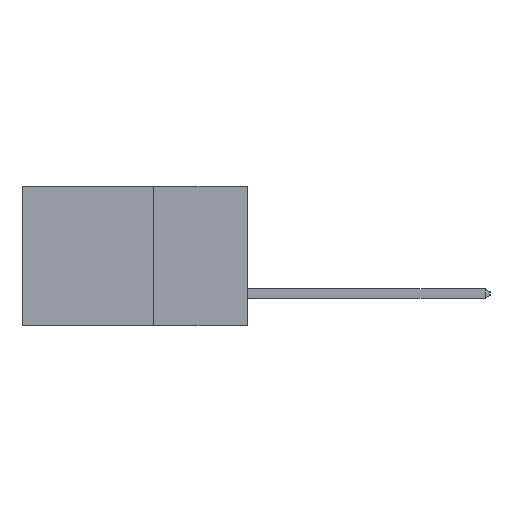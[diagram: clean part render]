
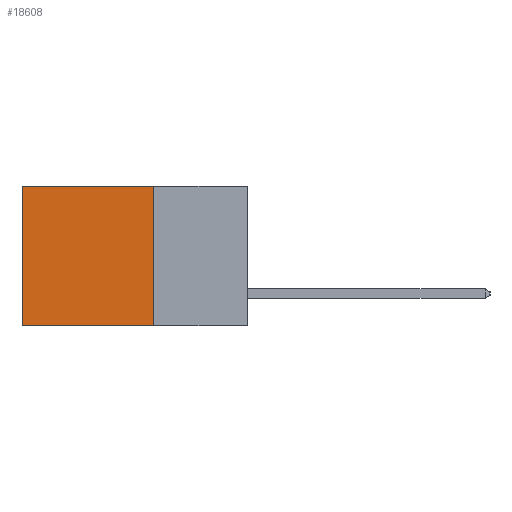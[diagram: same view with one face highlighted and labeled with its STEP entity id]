
A CAD part, left-side view. The second image highlights one B-rep face of the part: STEP entity #18608.
In plain terms, the highlighted planar face has unit normal (-1, 0, 0).
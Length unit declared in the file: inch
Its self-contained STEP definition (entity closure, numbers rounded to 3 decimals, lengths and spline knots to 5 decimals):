
#1206 = EDGE_LOOP ( 'NONE', ( #15318, #11464, #8101, #10656 ) ) ;
#1711 = CARTESIAN_POINT ( 'NONE',  ( 0.2615, 0.25, -0.37 ) ) ;
#1720 = DIRECTION ( 'NONE',  ( 0., 1., 0. ) ) ;
#1795 = VERTEX_POINT ( 'NONE', #19928 ) ;
#2093 = CARTESIAN_POINT ( 'NONE',  ( 0.2615, 0.25, 0. ) ) ;
#2266 = FACE_OUTER_BOUND ( 'NONE', #1206, .T. ) ;
#3436 = DIRECTION ( 'NONE',  ( 0., 0., -1. ) ) ;
#3667 = CARTESIAN_POINT ( 'NONE',  ( 0.2615, 0.25, -0.37 ) ) ;
#5673 = CARTESIAN_POINT ( 'NONE',  ( 0.2615, 0.6, -0.37 ) ) ;
#5714 = CARTESIAN_POINT ( 'NONE',  ( 0.2615, 0.6, 0. ) ) ;
#8101 = ORIENTED_EDGE ( 'NONE', *, *, #13003, .F. ) ;
#8709 = DIRECTION ( 'NONE',  ( 0., 1., 0. ) ) ;
#8888 = EDGE_CURVE ( 'NONE', #19064, #17308, #17690, .T. ) ;
#9465 = EDGE_CURVE ( 'NONE', #1795, #19064, #19101, .T. ) ;
#9545 = CARTESIAN_POINT ( 'NONE',  ( 0.2615, 0.25, -0.37 ) ) ;
#10656 = ORIENTED_EDGE ( 'NONE', *, *, #9465, .T. ) ;
#10678 = DIRECTION ( 'NONE',  ( 0., 0., -1. ) ) ;
#10701 = DIRECTION ( 'NONE',  ( 1., 0., 0. ) ) ;
#10753 = PLANE ( 'NONE',  #22346 ) ;
#10761 = CARTESIAN_POINT ( 'NONE',  ( 0.2615, 0.25, -0.37 ) ) ;
#11072 = VECTOR ( 'NONE', #8709, 39.37008 ) ;
#11464 = ORIENTED_EDGE ( 'NONE', *, *, #19765, .F. ) ;
#13003 = EDGE_CURVE ( 'NONE', #1795, #15977, #14561, .T. ) ;
#14561 = LINE ( 'NONE', #3667, #20723 ) ;
#15318 = ORIENTED_EDGE ( 'NONE', *, *, #8888, .T. ) ;
#15977 = VERTEX_POINT ( 'NONE', #1711 ) ;
#17308 = VERTEX_POINT ( 'NONE', #5673 ) ;
#17690 = LINE ( 'NONE', #22815, #22058 ) ;
#18608 = ADVANCED_FACE ( 'NONE', ( #2266 ), #10753, .F. ) ;
#19064 = VERTEX_POINT ( 'NONE', #5714 ) ;
#19101 = LINE ( 'NONE', #2093, #24015 ) ;
#19765 = EDGE_CURVE ( 'NONE', #15977, #17308, #21091, .T. ) ;
#19928 = CARTESIAN_POINT ( 'NONE',  ( 0.2615, 0.25, 0. ) ) ;
#20723 = VECTOR ( 'NONE', #3436, 39.37008 ) ;
#21091 = LINE ( 'NONE', #9545, #11072 ) ;
#22058 = VECTOR ( 'NONE', #23045, 39.37008 ) ;
#22346 = AXIS2_PLACEMENT_3D ( 'NONE', #10761, #10701, #10678 ) ;
#22815 = CARTESIAN_POINT ( 'NONE',  ( 0.2615, 0.6, -0.37 ) ) ;
#23045 = DIRECTION ( 'NONE',  ( 0., 0., -1. ) ) ;
#24015 = VECTOR ( 'NONE', #1720, 39.37008 ) ;
